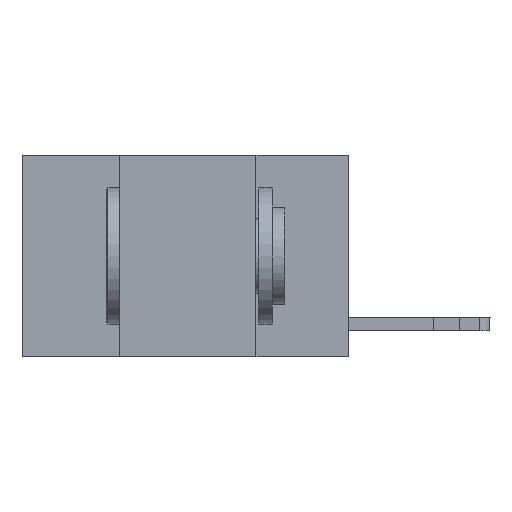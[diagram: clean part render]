
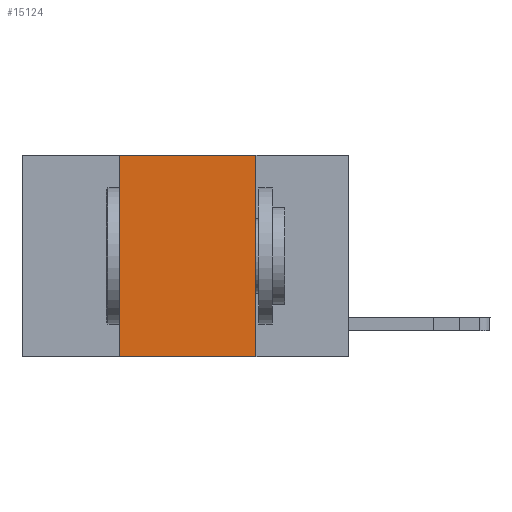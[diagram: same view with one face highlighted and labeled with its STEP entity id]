
A CAD part, left-side view. The second image highlights one B-rep face of the part: STEP entity #15124.
In plain terms, the highlighted planar face has unit normal (-1, 0, 0).
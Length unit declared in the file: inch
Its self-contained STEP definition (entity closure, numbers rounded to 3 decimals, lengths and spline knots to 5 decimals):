
#140 = CARTESIAN_POINT ( 'NONE',  ( 0., 0.17, 0. ) ) ;
#713 = FACE_OUTER_BOUND ( 'NONE', #17109, .T. ) ;
#759 = CARTESIAN_POINT ( 'NONE',  ( 0., 0.42, -0.37 ) ) ;
#774 = VECTOR ( 'NONE', #8223, 39.37008 ) ;
#1335 = LINE ( 'NONE', #5595, #5100 ) ;
#1367 = CARTESIAN_POINT ( 'NONE',  ( 0., 0.6, 0. ) ) ;
#1635 = EDGE_CURVE ( 'NONE', #3631, #7960, #1335, .T. ) ;
#1656 = DIRECTION ( 'NONE',  ( 0., 0., -1. ) ) ;
#1677 = CARTESIAN_POINT ( 'NONE',  ( 0., 0.17, -0.37 ) ) ;
#2234 = VECTOR ( 'NONE', #9837, 39.37008 ) ;
#2606 = EDGE_CURVE ( 'NONE', #3631, #10755, #6401, .T. ) ;
#2815 = DIRECTION ( 'NONE',  ( 0., -1., 0. ) ) ;
#3631 = VERTEX_POINT ( 'NONE', #759 ) ;
#4166 = CARTESIAN_POINT ( 'NONE',  ( 0., 0.42, 0. ) ) ;
#4468 = EDGE_CURVE ( 'NONE', #12858, #7960, #4563, .T. ) ;
#4563 = LINE ( 'NONE', #13539, #774 ) ;
#5100 = VECTOR ( 'NONE', #5556, 39.37008 ) ;
#5556 = DIRECTION ( 'NONE',  ( 0., -1., 0. ) ) ;
#5595 = CARTESIAN_POINT ( 'NONE',  ( 0., 0.6, -0.37 ) ) ;
#6336 = ORIENTED_EDGE ( 'NONE', *, *, #4468, .F. ) ;
#6401 = LINE ( 'NONE', #16288, #2234 ) ;
#7077 = ORIENTED_EDGE ( 'NONE', *, *, #14274, .F. ) ;
#7111 = ORIENTED_EDGE ( 'NONE', *, *, #1635, .T. ) ;
#7229 = PLANE ( 'NONE',  #15425 ) ;
#7960 = VERTEX_POINT ( 'NONE', #1677 ) ;
#8223 = DIRECTION ( 'NONE',  ( 0., 0., -1. ) ) ;
#8600 = CARTESIAN_POINT ( 'NONE',  ( 0., 0.6, 0. ) ) ;
#8660 = LINE ( 'NONE', #1367, #14440 ) ;
#9837 = DIRECTION ( 'NONE',  ( 0., 0., 1. ) ) ;
#9975 = DIRECTION ( 'NONE',  ( 1., 0., 0. ) ) ;
#10755 = VERTEX_POINT ( 'NONE', #4166 ) ;
#12858 = VERTEX_POINT ( 'NONE', #140 ) ;
#13539 = CARTESIAN_POINT ( 'NONE',  ( 0., 0.17, 0. ) ) ;
#14274 = EDGE_CURVE ( 'NONE', #10755, #12858, #8660, .T. ) ;
#14440 = VECTOR ( 'NONE', #2815, 39.37008 ) ;
#15100 = ORIENTED_EDGE ( 'NONE', *, *, #2606, .F. ) ;
#15124 = ADVANCED_FACE ( 'NONE', ( #713 ), #7229, .F. ) ;
#15425 = AXIS2_PLACEMENT_3D ( 'NONE', #8600, #9975, #1656 ) ;
#16288 = CARTESIAN_POINT ( 'NONE',  ( 0., 0.42, 0. ) ) ;
#17109 = EDGE_LOOP ( 'NONE', ( #6336, #7077, #15100, #7111 ) ) ;
